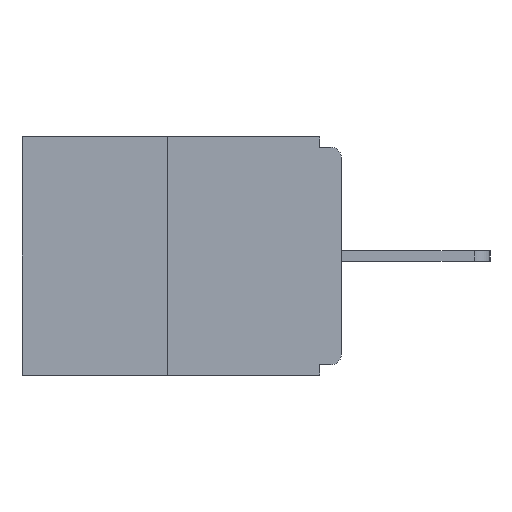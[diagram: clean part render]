
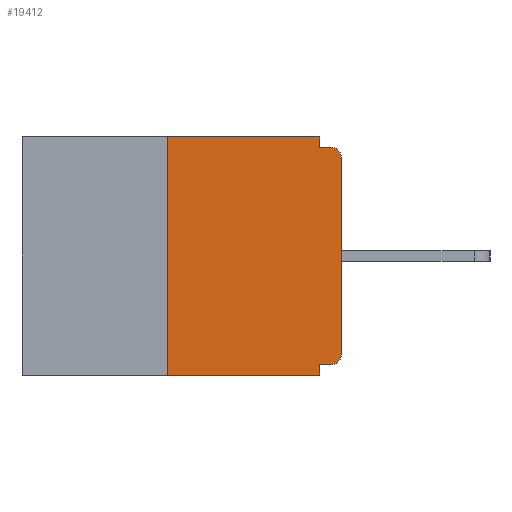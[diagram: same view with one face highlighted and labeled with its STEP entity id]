
A CAD part, left-side view. The second image highlights one B-rep face of the part: STEP entity #19412.
In plain terms, the highlighted planar face has unit normal (-1, 0, 0).
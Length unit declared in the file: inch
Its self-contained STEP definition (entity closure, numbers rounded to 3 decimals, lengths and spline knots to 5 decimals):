
#481 = DIRECTION ( 'NONE',  ( 0., -1., 0. ) ) ;
#1068 = CARTESIAN_POINT ( 'NONE',  ( 0., 0.46, 0. ) ) ;
#1130 = VERTEX_POINT ( 'NONE', #15357 ) ;
#2071 = EDGE_CURVE ( 'NONE', #6349, #6403, #14857, .T. ) ;
#2227 = CARTESIAN_POINT ( 'NONE',  ( 0., 0.015, -0.328 ) ) ;
#2393 = FACE_OUTER_BOUND ( 'NONE', #18559, .T. ) ;
#2704 = ORIENTED_EDGE ( 'NONE', *, *, #14492, .T. ) ;
#2739 = PLANE ( 'NONE',  #10718 ) ;
#3040 = EDGE_CURVE ( 'NONE', #10076, #8959, #7387, .T. ) ;
#3387 = DIRECTION ( 'NONE',  ( -1., 0., 0. ) ) ;
#3928 = ORIENTED_EDGE ( 'NONE', *, *, #5865, .T. ) ;
#4063 = LINE ( 'NONE', #7160, #18370 ) ;
#4671 = ORIENTED_EDGE ( 'NONE', *, *, #3040, .T. ) ;
#4740 = DIRECTION ( 'NONE',  ( 0., -1., 0. ) ) ;
#4778 = LINE ( 'NONE', #20582, #14236 ) ;
#4813 = VECTOR ( 'NONE', #11551, 39.37008 ) ;
#4887 = DIRECTION ( 'NONE',  ( 0., 0., 1. ) ) ;
#4933 = CARTESIAN_POINT ( 'NONE',  ( 0., 0.25, 0. ) ) ;
#5091 = CARTESIAN_POINT ( 'NONE',  ( 0., 0.015, -0.03 ) ) ;
#5455 = CIRCLE ( 'NONE', #21187, 0.015 ) ;
#5865 = EDGE_CURVE ( 'NONE', #9804, #6978, #14801, .T. ) ;
#5909 = ORIENTED_EDGE ( 'NONE', *, *, #12603, .F. ) ;
#6349 = VERTEX_POINT ( 'NONE', #10326 ) ;
#6403 = VERTEX_POINT ( 'NONE', #12046 ) ;
#6486 = VERTEX_POINT ( 'NONE', #11133 ) ;
#6978 = VERTEX_POINT ( 'NONE', #7048 ) ;
#7048 = CARTESIAN_POINT ( 'NONE',  ( 0., 0.015, -0.015 ) ) ;
#7160 = CARTESIAN_POINT ( 'NONE',  ( 0., 0.031, -0.343 ) ) ;
#7258 = DIRECTION ( 'NONE',  ( 0., 0., -1. ) ) ;
#7387 = LINE ( 'NONE', #17699, #8171 ) ;
#7712 = EDGE_CURVE ( 'NONE', #6403, #6978, #19947, .T. ) ;
#8171 = VECTOR ( 'NONE', #19861, 39.37008 ) ;
#8498 = VECTOR ( 'NONE', #10088, 39.37008 ) ;
#8515 = DIRECTION ( 'NONE',  ( -1., 0., 0. ) ) ;
#8907 = VERTEX_POINT ( 'NONE', #2227 ) ;
#8948 = EDGE_CURVE ( 'NONE', #1130, #8959, #4063, .T. ) ;
#8959 = VERTEX_POINT ( 'NONE', #12547 ) ;
#9039 = EDGE_CURVE ( 'NONE', #6486, #6349, #11613, .T. ) ;
#9321 = ORIENTED_EDGE ( 'NONE', *, *, #8948, .F. ) ;
#9384 = DIRECTION ( 'NONE',  ( 1., 0., 0. ) ) ;
#9804 = VERTEX_POINT ( 'NONE', #11428 ) ;
#9873 = LINE ( 'NONE', #4933, #8498 ) ;
#10076 = VERTEX_POINT ( 'NONE', #16076 ) ;
#10088 = DIRECTION ( 'NONE',  ( 0., 0., 1. ) ) ;
#10326 = CARTESIAN_POINT ( 'NONE',  ( 0., 0.031, 0. ) ) ;
#10718 = AXIS2_PLACEMENT_3D ( 'NONE', #14533, #9384, #16248 ) ;
#10817 = AXIS2_PLACEMENT_3D ( 'NONE', #5091, #8515, #7258 ) ;
#10903 = VECTOR ( 'NONE', #15093, 39.37008 ) ;
#11062 = DIRECTION ( 'NONE',  ( 0., 0., -1. ) ) ;
#11133 = CARTESIAN_POINT ( 'NONE',  ( 0., 0.25, 0. ) ) ;
#11428 = CARTESIAN_POINT ( 'NONE',  ( 0., 0., -0.03 ) ) ;
#11551 = DIRECTION ( 'NONE',  ( 0., 0., -1. ) ) ;
#11613 = LINE ( 'NONE', #1068, #13994 ) ;
#12009 = CARTESIAN_POINT ( 'NONE',  ( 0., 0., -0.328 ) ) ;
#12017 = VECTOR ( 'NONE', #481, 39.37008 ) ;
#12046 = CARTESIAN_POINT ( 'NONE',  ( 0., 0.031, -0.015 ) ) ;
#12547 = CARTESIAN_POINT ( 'NONE',  ( 0., 0.031, -0.343 ) ) ;
#12603 = EDGE_CURVE ( 'NONE', #8907, #1130, #15316, .T. ) ;
#13994 = VECTOR ( 'NONE', #4740, 39.37008 ) ;
#14236 = VECTOR ( 'NONE', #4887, 39.37008 ) ;
#14492 = EDGE_CURVE ( 'NONE', #21555, #9804, #4778, .T. ) ;
#14533 = CARTESIAN_POINT ( 'NONE',  ( 0., 0.46, 0. ) ) ;
#14548 = EDGE_CURVE ( 'NONE', #8907, #21555, #5455, .T. ) ;
#14801 = CIRCLE ( 'NONE', #10817, 0.015 ) ;
#14857 = LINE ( 'NONE', #21865, #4813 ) ;
#15093 = DIRECTION ( 'NONE',  ( 0., 1., 0. ) ) ;
#15316 = LINE ( 'NONE', #12009, #10903 ) ;
#15357 = CARTESIAN_POINT ( 'NONE',  ( 0., 0.031, -0.328 ) ) ;
#15750 = CARTESIAN_POINT ( 'NONE',  ( 0., 0.015, -0.313 ) ) ;
#15991 = ORIENTED_EDGE ( 'NONE', *, *, #7712, .F. ) ;
#16076 = CARTESIAN_POINT ( 'NONE',  ( 0., 0.25, -0.343 ) ) ;
#16182 = ORIENTED_EDGE ( 'NONE', *, *, #14548, .T. ) ;
#16248 = DIRECTION ( 'NONE',  ( 0., 0., -1. ) ) ;
#16378 = CARTESIAN_POINT ( 'NONE',  ( 0., 0., -0.015 ) ) ;
#17699 = CARTESIAN_POINT ( 'NONE',  ( 0., 0.46, -0.343 ) ) ;
#18370 = VECTOR ( 'NONE', #11062, 39.37008 ) ;
#18518 = ORIENTED_EDGE ( 'NONE', *, *, #9039, .F. ) ;
#18559 = EDGE_LOOP ( 'NONE', ( #18518, #22151, #4671, #9321, #5909, #16182, #2704, #3928, #15991, #19309 ) ) ;
#19179 = EDGE_CURVE ( 'NONE', #10076, #6486, #9873, .T. ) ;
#19309 = ORIENTED_EDGE ( 'NONE', *, *, #2071, .F. ) ;
#19412 = ADVANCED_FACE ( 'NONE', ( #2393 ), #2739, .F. ) ;
#19418 = DIRECTION ( 'NONE',  ( 0., 0., -1. ) ) ;
#19861 = DIRECTION ( 'NONE',  ( 0., -1., 0. ) ) ;
#19947 = LINE ( 'NONE', #16378, #12017 ) ;
#20434 = CARTESIAN_POINT ( 'NONE',  ( 0., 0., -0.313 ) ) ;
#20582 = CARTESIAN_POINT ( 'NONE',  ( 0., 0., 0. ) ) ;
#21187 = AXIS2_PLACEMENT_3D ( 'NONE', #15750, #3387, #19418 ) ;
#21555 = VERTEX_POINT ( 'NONE', #20434 ) ;
#21865 = CARTESIAN_POINT ( 'NONE',  ( 0., 0.031, 0. ) ) ;
#22151 = ORIENTED_EDGE ( 'NONE', *, *, #19179, .F. ) ;
